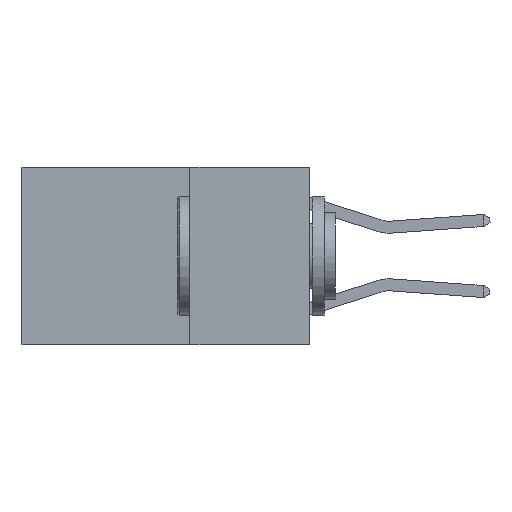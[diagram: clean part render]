
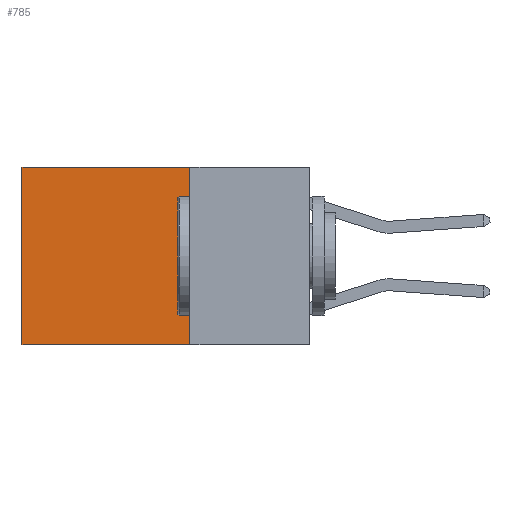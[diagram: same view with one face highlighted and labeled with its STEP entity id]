
A CAD part, left-side view. The second image highlights one B-rep face of the part: STEP entity #785.
In plain terms, the highlighted planar face has unit normal (-1, 0, 0).
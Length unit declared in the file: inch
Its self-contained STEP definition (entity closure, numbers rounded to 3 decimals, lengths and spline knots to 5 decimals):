
#306 = DIRECTION ( 'NONE',  ( 0., 0., -1. ) ) ;
#581 = VERTEX_POINT ( 'NONE', #7077 ) ;
#597 = PLANE ( 'NONE',  #7275 ) ;
#633 = VECTOR ( 'NONE', #10561, 39.37008 ) ;
#752 = ORIENTED_EDGE ( 'NONE', *, *, #4042, .F. ) ;
#785 = ADVANCED_FACE ( 'NONE', ( #4873 ), #597, .F. ) ;
#1422 = CARTESIAN_POINT ( 'NONE',  ( 0.2625, 0.25, 0. ) ) ;
#1518 = DIRECTION ( 'NONE',  ( 0., 1., 0. ) ) ;
#1776 = DIRECTION ( 'NONE',  ( 1., 0., 0. ) ) ;
#2312 = LINE ( 'NONE', #17234, #16919 ) ;
#2721 = CARTESIAN_POINT ( 'NONE',  ( 0.2625, 0.25, 0. ) ) ;
#4042 = EDGE_CURVE ( 'NONE', #581, #4621, #13737, .T. ) ;
#4621 = VERTEX_POINT ( 'NONE', #9245 ) ;
#4873 = FACE_OUTER_BOUND ( 'NONE', #12779, .T. ) ;
#5690 = VECTOR ( 'NONE', #6760, 39.37008 ) ;
#6463 = ORIENTED_EDGE ( 'NONE', *, *, #12374, .T. ) ;
#6760 = DIRECTION ( 'NONE',  ( 0., 0., -1. ) ) ;
#7077 = CARTESIAN_POINT ( 'NONE',  ( 0.2625, 0.25, -0.37 ) ) ;
#7275 = AXIS2_PLACEMENT_3D ( 'NONE', #13183, #1776, #10524 ) ;
#8065 = CARTESIAN_POINT ( 'NONE',  ( 0.2625, 0.25, 0. ) ) ;
#8111 = ORIENTED_EDGE ( 'NONE', *, *, #16547, .F. ) ;
#8113 = VECTOR ( 'NONE', #1518, 39.37008 ) ;
#9245 = CARTESIAN_POINT ( 'NONE',  ( 0.2625, 0.6, -0.37 ) ) ;
#10524 = DIRECTION ( 'NONE',  ( 0., 0., -1. ) ) ;
#10561 = DIRECTION ( 'NONE',  ( 0., 1., 0. ) ) ;
#10592 = LINE ( 'NONE', #2721, #8113 ) ;
#11483 = LINE ( 'NONE', #8065, #5690 ) ;
#11692 = VERTEX_POINT ( 'NONE', #1422 ) ;
#11896 = EDGE_CURVE ( 'NONE', #12066, #4621, #2312, .T. ) ;
#12066 = VERTEX_POINT ( 'NONE', #17669 ) ;
#12220 = ORIENTED_EDGE ( 'NONE', *, *, #11896, .T. ) ;
#12374 = EDGE_CURVE ( 'NONE', #11692, #12066, #10592, .T. ) ;
#12779 = EDGE_LOOP ( 'NONE', ( #12220, #752, #8111, #6463 ) ) ;
#13183 = CARTESIAN_POINT ( 'NONE',  ( 0.2625, 0.25, 0. ) ) ;
#13737 = LINE ( 'NONE', #17626, #633 ) ;
#16547 = EDGE_CURVE ( 'NONE', #11692, #581, #11483, .T. ) ;
#16919 = VECTOR ( 'NONE', #306, 39.37008 ) ;
#17234 = CARTESIAN_POINT ( 'NONE',  ( 0.2625, 0.6, 0. ) ) ;
#17626 = CARTESIAN_POINT ( 'NONE',  ( 0.2625, 0.25, -0.37 ) ) ;
#17669 = CARTESIAN_POINT ( 'NONE',  ( 0.2625, 0.6, 0. ) ) ;
